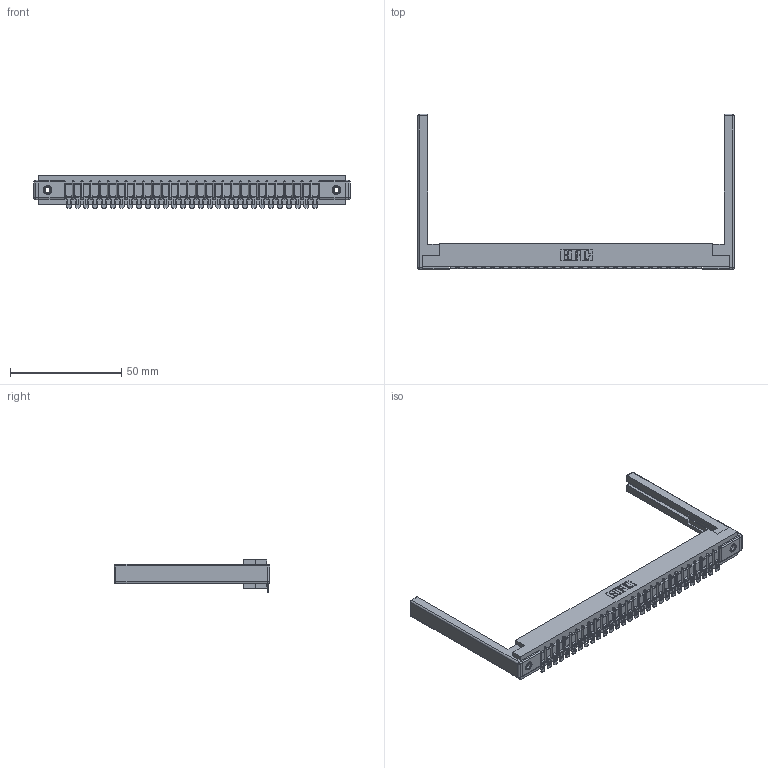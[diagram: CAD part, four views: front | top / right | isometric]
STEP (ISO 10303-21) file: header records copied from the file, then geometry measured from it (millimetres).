
FILE_DESCRIPTION (( 'STEP AP203' ), '1' );
FILE_NAME ('357-029-454-168.STEP', '2020-10-02T00:02:59', ( '' ), ( '' ), 'SwSTEP 2.0', 'SolidWorks 2020', '' );
FILE_SCHEMA (( 'CONFIG_CONTROL_DESIGN' ));
Length unit declared in the file: inch
Products named in the file (5): 345-250-001_345-250-001-102; 307-220-068; 357-029-454-168; 307-290-002_554; 307 Part_.156 Dia Mounting Holes
Assembly tree (34 placements, depth 2):
  357-029-454-168
    307 Part_.156 Dia Mounting Holes
    307-290-002_554  x29
    307-220-068  x2
    345-250-001_345-250-001-102  x2
Bounding box: 142.34 x 69.98 x 14.52 mm (x, y, z)
Volume: 19523.5 mm3; surface area: 22832 mm2
Topology: 34 solids, 34 shells, 2651 faces, 8050 edges, 5264 vertices
Faces by surface type: plane 1492, cylinder 1075, sphere 68, cone 12, torus 4
Entity records: 30188 total; most frequent: CARTESIAN_POINT 5055, ORIENTED_EDGE 5034, DIRECTION 4941, EDGE_CURVE 2517, VECTOR 1913, LINE 1913, VERTEX_POINT 1628, AXIS2_PLACEMENT_3D 1514
